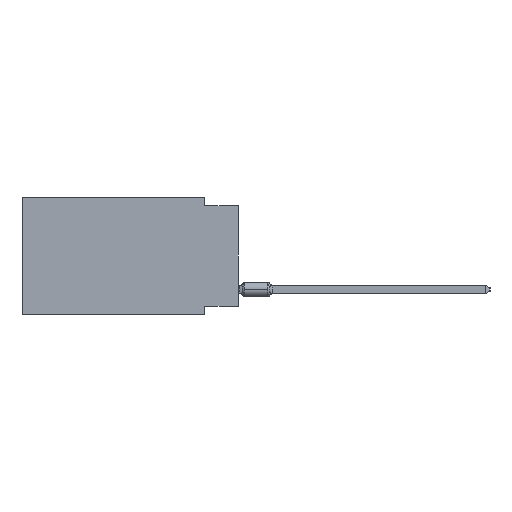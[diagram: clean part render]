
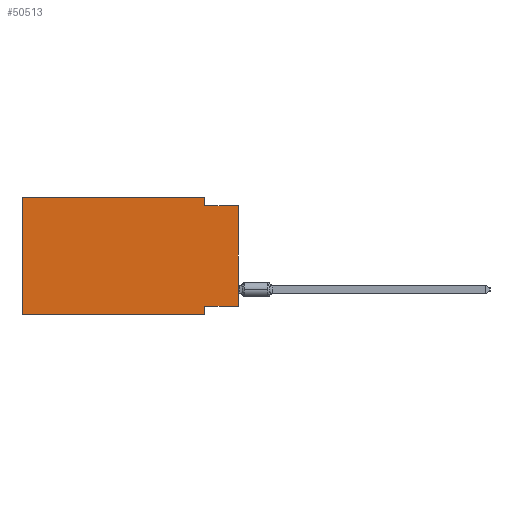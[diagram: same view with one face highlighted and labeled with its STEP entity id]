
A CAD part, left-side view. The second image highlights one B-rep face of the part: STEP entity #50513.
In plain terms, the highlighted planar face has unit normal (-1, 0, 0).
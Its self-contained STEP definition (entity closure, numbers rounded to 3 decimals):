
#76 = LINE ( 'NONE', #47223, #18224 ) ;
#817 = DIRECTION ( 'NONE',  ( 1., 0., 0. ) ) ;
#1016 = AXIS2_PLACEMENT_3D ( 'NONE', #40276, #817, #44432 ) ;
#1060 = CARTESIAN_POINT ( 'NONE',  ( 0., 16.383, -8.89 ) ) ;
#4048 = ORIENTED_EDGE ( 'NONE', *, *, #9700, .F. ) ;
#4822 = ORIENTED_EDGE ( 'NONE', *, *, #43197, .F. ) ;
#4961 = VERTEX_POINT ( 'NONE', #12656 ) ;
#7163 = PLANE ( 'NONE',  #1016 ) ;
#7911 = CARTESIAN_POINT ( 'NONE',  ( 0., 0., -0.635 ) ) ;
#7948 = EDGE_LOOP ( 'NONE', ( #13905, #29369, #4048, #18714, #26275, #29597, #32677, #4822 ) ) ;
#8057 = VECTOR ( 'NONE', #53856, 1000. ) ;
#8651 = DIRECTION ( 'NONE',  ( 0., 0., -1. ) ) ;
#8704 = CARTESIAN_POINT ( 'NONE',  ( 0., 2.54, -8.89 ) ) ;
#9203 = VERTEX_POINT ( 'NONE', #12155 ) ;
#9288 = LINE ( 'NONE', #14684, #26109 ) ;
#9700 = EDGE_CURVE ( 'NONE', #9203, #61981, #41991, .T. ) ;
#10634 = CARTESIAN_POINT ( 'NONE',  ( 0., 0., 0. ) ) ;
#10791 = VECTOR ( 'NONE', #8651, 1000. ) ;
#12155 = CARTESIAN_POINT ( 'NONE',  ( 0., 2.54, 0. ) ) ;
#12383 = VECTOR ( 'NONE', #15331, 1000. ) ;
#12470 = LINE ( 'NONE', #31889, #35038 ) ;
#12656 = CARTESIAN_POINT ( 'NONE',  ( 0., 0., -8.255 ) ) ;
#13674 = VERTEX_POINT ( 'NONE', #7911 ) ;
#13905 = ORIENTED_EDGE ( 'NONE', *, *, #52104, .T. ) ;
#14684 = CARTESIAN_POINT ( 'NONE',  ( 0., 16.383, 0. ) ) ;
#15331 = DIRECTION ( 'NONE',  ( 0., -1., 0. ) ) ;
#15573 = VERTEX_POINT ( 'NONE', #36827 ) ;
#16707 = FACE_OUTER_BOUND ( 'NONE', #7948, .T. ) ;
#16977 = VERTEX_POINT ( 'NONE', #51844 ) ;
#18224 = VECTOR ( 'NONE', #23952, 1000. ) ;
#18714 = ORIENTED_EDGE ( 'NONE', *, *, #54679, .F. ) ;
#21110 = LINE ( 'NONE', #10634, #27631 ) ;
#23952 = DIRECTION ( 'NONE',  ( 0., -1., 0. ) ) ;
#24320 = VERTEX_POINT ( 'NONE', #8704 ) ;
#24453 = VERTEX_POINT ( 'NONE', #1060 ) ;
#24731 = EDGE_CURVE ( 'NONE', #15573, #24320, #43646, .T. ) ;
#26109 = VECTOR ( 'NONE', #48124, 1000. ) ;
#26275 = ORIENTED_EDGE ( 'NONE', *, *, #37355, .F. ) ;
#27631 = VECTOR ( 'NONE', #36068, 1000. ) ;
#28440 = EDGE_CURVE ( 'NONE', #61981, #13674, #76, .T. ) ;
#29369 = ORIENTED_EDGE ( 'NONE', *, *, #28440, .F. ) ;
#29597 = ORIENTED_EDGE ( 'NONE', *, *, #45840, .T. ) ;
#31889 = CARTESIAN_POINT ( 'NONE',  ( 0., 0., -8.255 ) ) ;
#32677 = ORIENTED_EDGE ( 'NONE', *, *, #24731, .F. ) ;
#32978 = CARTESIAN_POINT ( 'NONE',  ( 0., 2.54, -0.635 ) ) ;
#34426 = CARTESIAN_POINT ( 'NONE',  ( 0., 16.383, 0. ) ) ;
#35038 = VECTOR ( 'NONE', #51308, 1000. ) ;
#35057 = CARTESIAN_POINT ( 'NONE',  ( 0., 16.383, -8.89 ) ) ;
#36068 = DIRECTION ( 'NONE',  ( 0., 0., 1. ) ) ;
#36827 = CARTESIAN_POINT ( 'NONE',  ( 0., 2.54, -8.255 ) ) ;
#37355 = EDGE_CURVE ( 'NONE', #24453, #16977, #49078, .T. ) ;
#40276 = CARTESIAN_POINT ( 'NONE',  ( 0., 16.383, 0. ) ) ;
#41991 = LINE ( 'NONE', #61111, #54715 ) ;
#43197 = EDGE_CURVE ( 'NONE', #4961, #15573, #12470, .T. ) ;
#43646 = LINE ( 'NONE', #57056, #10791 ) ;
#44432 = DIRECTION ( 'NONE',  ( 0., 0., -1. ) ) ;
#45840 = EDGE_CURVE ( 'NONE', #24453, #24320, #54178, .T. ) ;
#46769 = DIRECTION ( 'NONE',  ( 0., 0., -1. ) ) ;
#47223 = CARTESIAN_POINT ( 'NONE',  ( 0., 0., -0.635 ) ) ;
#48124 = DIRECTION ( 'NONE',  ( 0., -1., 0. ) ) ;
#49078 = LINE ( 'NONE', #34426, #8057 ) ;
#50513 = ADVANCED_FACE ( 'NONE', ( #16707 ), #7163, .F. ) ;
#51308 = DIRECTION ( 'NONE',  ( 0., 1., 0. ) ) ;
#51844 = CARTESIAN_POINT ( 'NONE',  ( 0., 16.383, 0. ) ) ;
#52104 = EDGE_CURVE ( 'NONE', #4961, #13674, #21110, .T. ) ;
#53856 = DIRECTION ( 'NONE',  ( 0., 0., 1. ) ) ;
#54178 = LINE ( 'NONE', #35057, #12383 ) ;
#54679 = EDGE_CURVE ( 'NONE', #16977, #9203, #9288, .T. ) ;
#54715 = VECTOR ( 'NONE', #46769, 1000. ) ;
#57056 = CARTESIAN_POINT ( 'NONE',  ( 0., 2.54, -8.89 ) ) ;
#61111 = CARTESIAN_POINT ( 'NONE',  ( 0., 2.54, 0. ) ) ;
#61981 = VERTEX_POINT ( 'NONE', #32978 ) ;
